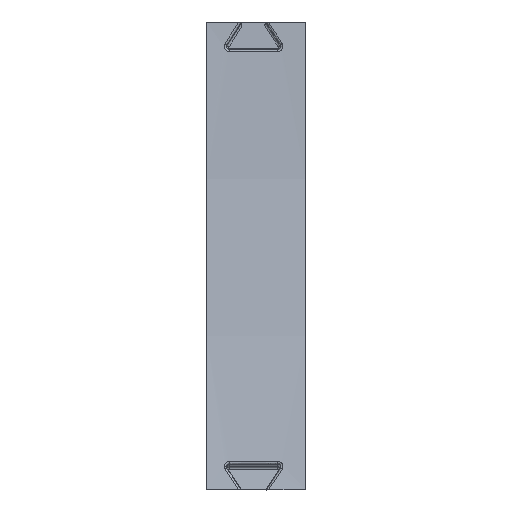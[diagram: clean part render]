
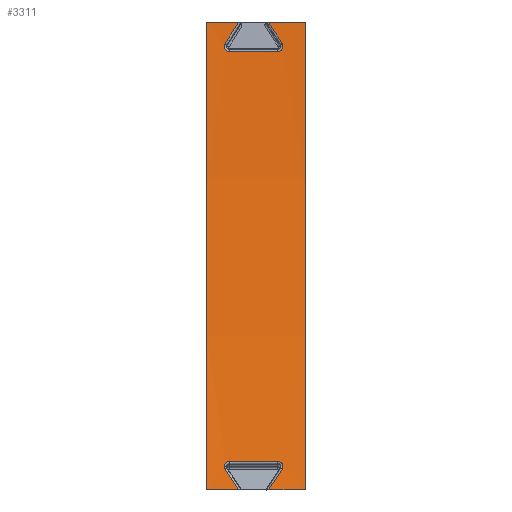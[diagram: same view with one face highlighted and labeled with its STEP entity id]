
A CAD part, left-side view. The second image highlights one B-rep face of the part: STEP entity #3311.
In plain terms, the highlighted cylindrical face has radius 949 mm (diameter 1898 mm), a partial arc.
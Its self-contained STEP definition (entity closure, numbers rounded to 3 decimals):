
#38=B_SPLINE_CURVE_WITH_KNOTS('',3,(#5084,#5085,#5086,#5087,#5088,#5089,
#5090),.UNSPECIFIED.,.F.,.F.,(4,1,1,1,4),(-0.373,-0.293,
-0.213,-0.106,0.),
 .UNSPECIFIED.);
#40=B_SPLINE_CURVE_WITH_KNOTS('',3,(#5121,#5122,#5123,#5124),
 .UNSPECIFIED.,.F.,.F.,(4,4),(-0.82,0.82),
 .UNSPECIFIED.);
#42=B_SPLINE_CURVE_WITH_KNOTS('',3,(#5167,#5168,#5169,#5170,#5171,#5172,
#5173),.UNSPECIFIED.,.F.,.F.,(4,1,1,1,4),(-0.373,-0.266,
-0.16,-0.08,0.),
 .UNSPECIFIED.);
#47=B_SPLINE_CURVE_WITH_KNOTS('',3,(#5240,#5241,#5242,#5243),
 .UNSPECIFIED.,.F.,.F.,(4,4),(-2.307,-2.199),
 .UNSPECIFIED.);
#48=B_SPLINE_CURVE_WITH_KNOTS('',3,(#5245,#5246,#5247,#5248,#5249),
 .UNSPECIFIED.,.F.,.F.,(4,1,4),(-1.1,-0.987,-0.836),
 .UNSPECIFIED.);
#49=B_SPLINE_CURVE_WITH_KNOTS('',3,(#5251,#5252,#5253,#5254),
 .UNSPECIFIED.,.F.,.F.,(4,4),(-0.82,0.82),
 .UNSPECIFIED.);
#50=B_SPLINE_CURVE_WITH_KNOTS('',3,(#5256,#5257,#5258,#5259,#5260,#5261,
#5262),.UNSPECIFIED.,.F.,.F.,(4,1,1,1,4),(-0.373,-0.266,
-0.16,-0.08,0.),
 .UNSPECIFIED.);
#226=FACE_OUTER_BOUND('',#435,.T.);
#435=EDGE_LOOP('',(#2217,#2218,#2219,#2220,#2221,#2222,#2223,#2224,#2225,
#2226,#2227,#2228,#2229,#2230,#2231,#2232,#2233));
#635=ELLIPSE('',#3538,1119.255,949.);
#636=ELLIPSE('',#3542,1119.289,949.);
#638=ELLIPSE('',#3547,1119.289,949.);
#639=ELLIPSE('',#3548,1119.289,949.);
#697=LINE('',#5232,#916);
#698=LINE('',#5236,#917);
#699=LINE('',#5266,#918);
#700=LINE('',#5269,#919);
#916=VECTOR('',#3979,10.);
#917=VECTOR('',#3982,10.);
#918=VECTOR('',#3987,10.);
#919=VECTOR('',#3990,10.);
#1135=CIRCLE('',#3546,949.);
#1136=CIRCLE('',#3549,949.);
#1327=VERTEX_POINT('',#5032);
#1328=VERTEX_POINT('',#5034);
#1330=VERTEX_POINT('',#5082);
#1332=VERTEX_POINT('',#5119);
#1334=VERTEX_POINT('',#5165);
#1336=VERTEX_POINT('',#5202);
#1339=VERTEX_POINT('',#5231);
#1340=VERTEX_POINT('',#5233);
#1341=VERTEX_POINT('',#5235);
#1342=VERTEX_POINT('',#5237);
#1343=VERTEX_POINT('',#5239);
#1344=VERTEX_POINT('',#5244);
#1345=VERTEX_POINT('',#5250);
#1346=VERTEX_POINT('',#5255);
#1347=VERTEX_POINT('',#5263);
#1348=VERTEX_POINT('',#5265);
#1349=VERTEX_POINT('',#5267);
#1654=EDGE_CURVE('',#1327,#1328,#635,.T.);
#1657=EDGE_CURVE('',#1330,#1327,#38,.T.);
#1660=EDGE_CURVE('',#1332,#1330,#40,.T.);
#1663=EDGE_CURVE('',#1334,#1332,#42,.T.);
#1666=EDGE_CURVE('',#1336,#1334,#636,.T.);
#1672=EDGE_CURVE('',#1339,#1336,#697,.T.);
#1673=EDGE_CURVE('',#1339,#1340,#1135,.T.);
#1674=EDGE_CURVE('',#1340,#1341,#698,.T.);
#1675=EDGE_CURVE('',#1342,#1341,#638,.T.);
#1676=EDGE_CURVE('',#1343,#1342,#47,.T.);
#1677=EDGE_CURVE('',#1344,#1343,#48,.T.);
#1678=EDGE_CURVE('',#1345,#1344,#49,.T.);
#1679=EDGE_CURVE('',#1346,#1345,#50,.T.);
#1680=EDGE_CURVE('',#1347,#1346,#639,.T.);
#1681=EDGE_CURVE('',#1347,#1348,#699,.T.);
#1682=EDGE_CURVE('',#1349,#1348,#1136,.T.);
#1683=EDGE_CURVE('',#1328,#1349,#700,.T.);
#2217=ORIENTED_EDGE('',*,*,#1654,.F.);
#2218=ORIENTED_EDGE('',*,*,#1657,.F.);
#2219=ORIENTED_EDGE('',*,*,#1660,.F.);
#2220=ORIENTED_EDGE('',*,*,#1663,.F.);
#2221=ORIENTED_EDGE('',*,*,#1666,.F.);
#2222=ORIENTED_EDGE('',*,*,#1672,.F.);
#2223=ORIENTED_EDGE('',*,*,#1673,.T.);
#2224=ORIENTED_EDGE('',*,*,#1674,.T.);
#2225=ORIENTED_EDGE('',*,*,#1675,.F.);
#2226=ORIENTED_EDGE('',*,*,#1676,.F.);
#2227=ORIENTED_EDGE('',*,*,#1677,.F.);
#2228=ORIENTED_EDGE('',*,*,#1678,.F.);
#2229=ORIENTED_EDGE('',*,*,#1679,.F.);
#2230=ORIENTED_EDGE('',*,*,#1680,.F.);
#2231=ORIENTED_EDGE('',*,*,#1681,.T.);
#2232=ORIENTED_EDGE('',*,*,#1682,.F.);
#2233=ORIENTED_EDGE('',*,*,#1683,.F.);
#3221=CYLINDRICAL_SURFACE('',#3545,949.);
#3311=ADVANCED_FACE('',(#226),#3221,.F.);
#3538=AXIS2_PLACEMENT_3D('',#5035,#3961,#3962);
#3542=AXIS2_PLACEMENT_3D('',#5215,#3969,#3970);
#3545=AXIS2_PLACEMENT_3D('',#5230,#3977,#3978);
#3546=AXIS2_PLACEMENT_3D('',#5234,#3980,#3981);
#3547=AXIS2_PLACEMENT_3D('',#5238,#3983,#3984);
#3548=AXIS2_PLACEMENT_3D('',#5264,#3985,#3986);
#3549=AXIS2_PLACEMENT_3D('',#5268,#3988,#3989);
#3961=DIRECTION('center_axis',(0.046,-0.848,0.528));
#3962=DIRECTION('ref_axis',(-0.074,-0.53,-0.845));
#3969=DIRECTION('center_axis',(0.046,0.848,0.528));
#3970=DIRECTION('ref_axis',(-0.074,0.53,-0.845));
#3977=DIRECTION('center_axis',(0.,1.,0.));
#3978=DIRECTION('ref_axis',(1.,0.,-0.031));
#3979=DIRECTION('',(0.,-1.,0.));
#3980=DIRECTION('center_axis',(0.,1.,0.));
#3981=DIRECTION('ref_axis',(1.,0.,-0.031));
#3982=DIRECTION('',(0.,-1.,0.));
#3983=DIRECTION('center_axis',(-0.137,0.848,-0.512));
#3984=DIRECTION('ref_axis',(0.219,0.53,0.819));
#3985=DIRECTION('center_axis',(-0.137,-0.848,-0.512));
#3986=DIRECTION('ref_axis',(0.219,-0.53,0.819));
#3987=DIRECTION('',(0.,-1.,0.));
#3988=DIRECTION('center_axis',(0.,1.,0.));
#3989=DIRECTION('ref_axis',(1.,0.,-0.031));
#3990=DIRECTION('',(0.,-1.,0.));
#5032=CARTESIAN_POINT('',(-104.48,14.069,-88.663));
#5034=CARTESIAN_POINT('',(-103.794,18.671,-81.334));
#5035=CARTESIAN_POINT('Origin',(-1048.998,19.987,3.472));
#5082=CARTESIAN_POINT('',(-104.744,15.552,-91.325));
#5084=CARTESIAN_POINT('Ctrl Pts',(-104.744,15.552,-91.325));
#5085=CARTESIAN_POINT('Ctrl Pts',(-104.744,15.286,-91.325));
#5086=CARTESIAN_POINT('Ctrl Pts',(-104.731,14.755,-91.202));
#5087=CARTESIAN_POINT('Ctrl Pts',(-104.674,14.048,-90.63));
#5088=CARTESIAN_POINT('Ctrl Pts',(-104.58,13.694,-89.677));
#5089=CARTESIAN_POINT('Ctrl Pts',(-104.509,13.881,-88.962));
#5090=CARTESIAN_POINT('Ctrl Pts',(-104.48,14.069,-88.663));
#5119=CARTESIAN_POINT('',(-104.745,31.944,-91.333));
#5121=CARTESIAN_POINT('Ctrl Pts',(-104.745,31.944,-91.333));
#5122=CARTESIAN_POINT('Ctrl Pts',(-104.744,26.48,-91.33));
#5123=CARTESIAN_POINT('Ctrl Pts',(-104.744,21.016,-91.328));
#5124=CARTESIAN_POINT('Ctrl Pts',(-104.744,15.552,-91.325));
#5165=CARTESIAN_POINT('',(-104.481,33.429,-88.67));
#5167=CARTESIAN_POINT('Ctrl Pts',(-104.481,33.429,-88.67));
#5168=CARTESIAN_POINT('Ctrl Pts',(-104.51,33.617,-88.97));
#5169=CARTESIAN_POINT('Ctrl Pts',(-104.58,33.804,-89.686));
#5170=CARTESIAN_POINT('Ctrl Pts',(-104.675,33.449,-90.638));
#5171=CARTESIAN_POINT('Ctrl Pts',(-104.732,32.742,-91.21));
#5172=CARTESIAN_POINT('Ctrl Pts',(-104.745,32.21,-91.333));
#5173=CARTESIAN_POINT('Ctrl Pts',(-104.745,31.944,-91.333));
#5202=CARTESIAN_POINT('',(-103.794,28.821,-81.334));
#5215=CARTESIAN_POINT('Origin',(-1048.998,27.505,3.472));
#5230=CARTESIAN_POINT('Origin',(-1048.998,22.926,3.472));
#5231=CARTESIAN_POINT('',(-103.794,39.734,-81.334));
#5232=CARTESIAN_POINT('',(-103.794,22.926,-81.334));
#5233=CARTESIAN_POINT('',(-131.781,39.734,-240.077));
#5234=CARTESIAN_POINT('Origin',(-1048.998,39.734,3.472));
#5235=CARTESIAN_POINT('',(-131.781,28.85,-240.077));
#5236=CARTESIAN_POINT('',(-131.781,22.926,-240.077));
#5237=CARTESIAN_POINT('',(-129.929,33.429,-232.992));
#5238=CARTESIAN_POINT('Origin',(-1048.998,27.51,3.472));
#5239=CARTESIAN_POINT('',(-129.673,33.692,-231.994));
#5240=CARTESIAN_POINT('Ctrl Pts',(-129.673,33.692,-231.994));
#5241=CARTESIAN_POINT('Ctrl Pts',(-129.762,33.713,-232.342));
#5242=CARTESIAN_POINT('Ctrl Pts',(-129.853,33.62,-232.696));
#5243=CARTESIAN_POINT('Ctrl Pts',(-129.929,33.429,-232.992));
#5244=CARTESIAN_POINT('',(-129.269,31.947,-230.409));
#5245=CARTESIAN_POINT('Ctrl Pts',(-129.269,31.947,-230.409));
#5246=CARTESIAN_POINT('Ctrl Pts',(-129.269,32.323,-230.409));
#5247=CARTESIAN_POINT('Ctrl Pts',(-129.341,33.202,-230.693));
#5248=CARTESIAN_POINT('Ctrl Pts',(-129.549,33.66,-231.509));
#5249=CARTESIAN_POINT('Ctrl Pts',(-129.673,33.692,-231.994));
#5250=CARTESIAN_POINT('',(-129.267,15.555,-230.401));
#5251=CARTESIAN_POINT('Ctrl Pts',(-129.267,15.555,-230.401));
#5252=CARTESIAN_POINT('Ctrl Pts',(-129.267,21.019,-230.403));
#5253=CARTESIAN_POINT('Ctrl Pts',(-129.268,26.483,-230.406));
#5254=CARTESIAN_POINT('Ctrl Pts',(-129.269,31.947,-230.409));
#5255=CARTESIAN_POINT('',(-129.93,14.07,-232.993));
#5256=CARTESIAN_POINT('Ctrl Pts',(-129.93,14.07,-232.993));
#5257=CARTESIAN_POINT('Ctrl Pts',(-129.855,13.882,-232.701));
#5258=CARTESIAN_POINT('Ctrl Pts',(-129.676,13.695,-232.005));
#5259=CARTESIAN_POINT('Ctrl Pts',(-129.439,14.05,-231.077));
#5260=CARTESIAN_POINT('Ctrl Pts',(-129.297,14.757,-230.52));
#5261=CARTESIAN_POINT('Ctrl Pts',(-129.267,15.289,-230.401));
#5262=CARTESIAN_POINT('Ctrl Pts',(-129.267,15.555,-230.401));
#5263=CARTESIAN_POINT('',(-131.781,18.649,-240.077));
#5264=CARTESIAN_POINT('Origin',(-1048.998,19.989,3.472));
#5265=CARTESIAN_POINT('',(-131.781,6.118,-240.077));
#5266=CARTESIAN_POINT('',(-131.781,22.926,-240.077));
#5267=CARTESIAN_POINT('',(-103.794,6.118,-81.334));
#5268=CARTESIAN_POINT('Origin',(-1048.998,6.118,3.472));
#5269=CARTESIAN_POINT('',(-103.794,22.926,-81.334));
